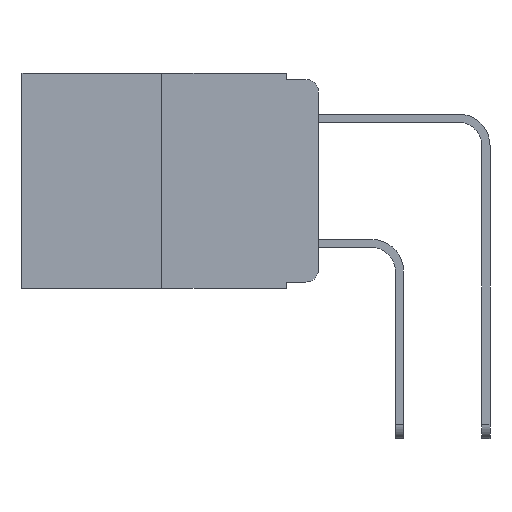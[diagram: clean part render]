
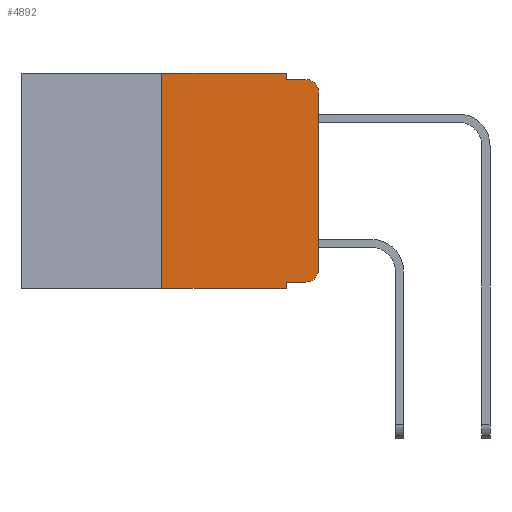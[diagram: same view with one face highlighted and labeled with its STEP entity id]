
A CAD part, left-side view. The second image highlights one B-rep face of the part: STEP entity #4892.
In plain terms, the highlighted planar face has unit normal (-1, 0, 0).
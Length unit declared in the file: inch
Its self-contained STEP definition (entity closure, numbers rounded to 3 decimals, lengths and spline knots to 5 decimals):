
#120 = LINE ( 'NONE', #3760, #2775 ) ;
#533 = VERTEX_POINT ( 'NONE', #3398 ) ;
#563 = EDGE_CURVE ( 'NONE', #5726, #13328, #4912, .T. ) ;
#716 = AXIS2_PLACEMENT_3D ( 'NONE', #894, #8579, #2016 ) ;
#840 = ORIENTED_EDGE ( 'NONE', *, *, #13257, .F. ) ;
#894 = CARTESIAN_POINT ( 'NONE',  ( 0., 0.02, -0.313 ) ) ;
#1143 = DIRECTION ( 'NONE',  ( 0., 0., -1. ) ) ;
#1167 = CARTESIAN_POINT ( 'NONE',  ( 0., 0.02, -0.01 ) ) ;
#1202 = AXIS2_PLACEMENT_3D ( 'NONE', #4929, #8517, #8490 ) ;
#1259 = ORIENTED_EDGE ( 'NONE', *, *, #12910, .F. ) ;
#1360 = VECTOR ( 'NONE', #7887, 39.37008 ) ;
#1500 = VERTEX_POINT ( 'NONE', #2942 ) ;
#1526 = FACE_OUTER_BOUND ( 'NONE', #5197, .T. ) ;
#1899 = EDGE_CURVE ( 'NONE', #3154, #9346, #120, .T. ) ;
#2016 = DIRECTION ( 'NONE',  ( 0., 0., -1. ) ) ;
#2288 = EDGE_CURVE ( 'NONE', #3154, #12996, #7619, .T. ) ;
#2687 = CARTESIAN_POINT ( 'NONE',  ( 0., 0., -0.03 ) ) ;
#2737 = CARTESIAN_POINT ( 'NONE',  ( 0., 0.02, -0.333 ) ) ;
#2763 = ORIENTED_EDGE ( 'NONE', *, *, #1899, .F. ) ;
#2775 = VECTOR ( 'NONE', #8216, 39.37008 ) ;
#2942 = CARTESIAN_POINT ( 'NONE',  ( 0., 0.051, 0. ) ) ;
#3154 = VERTEX_POINT ( 'NONE', #10959 ) ;
#3174 = VERTEX_POINT ( 'NONE', #12846 ) ;
#3245 = LINE ( 'NONE', #8955, #5864 ) ;
#3398 = CARTESIAN_POINT ( 'NONE',  ( 0., 0., -0.313 ) ) ;
#3599 = DIRECTION ( 'NONE',  ( 0., -1., 0. ) ) ;
#3760 = CARTESIAN_POINT ( 'NONE',  ( 0., 0.051, 0. ) ) ;
#3781 = CARTESIAN_POINT ( 'NONE',  ( 0., 0.25, -0.343 ) ) ;
#4087 = VERTEX_POINT ( 'NONE', #9158 ) ;
#4281 = EDGE_CURVE ( 'NONE', #8876, #3174, #3245, .T. ) ;
#4892 = ADVANCED_FACE ( 'NONE', ( #1526 ), #13605, .F. ) ;
#4912 = CIRCLE ( 'NONE', #10107, 0.02 ) ;
#4929 = CARTESIAN_POINT ( 'NONE',  ( 0., 0.473, 0. ) ) ;
#5197 = EDGE_LOOP ( 'NONE', ( #13562, #7465, #7934, #1259, #840, #12431, #11138, #2763, #11366, #8012 ) ) ;
#5726 = VERTEX_POINT ( 'NONE', #2687 ) ;
#5864 = VECTOR ( 'NONE', #13428, 39.37008 ) ;
#6359 = CARTESIAN_POINT ( 'NONE',  ( 0., 0.051, -0.01 ) ) ;
#6771 = LINE ( 'NONE', #8696, #8895 ) ;
#6962 = CIRCLE ( 'NONE', #716, 0.02 ) ;
#7018 = LINE ( 'NONE', #6359, #12185 ) ;
#7078 = DIRECTION ( 'NONE',  ( 0., -1., 0. ) ) ;
#7273 = VECTOR ( 'NONE', #3599, 39.37008 ) ;
#7463 = DIRECTION ( 'NONE',  ( 0., -1., 0. ) ) ;
#7465 = ORIENTED_EDGE ( 'NONE', *, *, #563, .T. ) ;
#7619 = LINE ( 'NONE', #13013, #7273 ) ;
#7887 = DIRECTION ( 'NONE',  ( 0., 0., 1. ) ) ;
#7934 = ORIENTED_EDGE ( 'NONE', *, *, #10855, .F. ) ;
#7939 = VECTOR ( 'NONE', #13244, 39.37008 ) ;
#8012 = ORIENTED_EDGE ( 'NONE', *, *, #12567, .T. ) ;
#8216 = DIRECTION ( 'NONE',  ( 0., 0., -1. ) ) ;
#8268 = EDGE_CURVE ( 'NONE', #8876, #9346, #12326, .T. ) ;
#8490 = DIRECTION ( 'NONE',  ( 0., 0., -1. ) ) ;
#8517 = DIRECTION ( 'NONE',  ( 1., 0., 0. ) ) ;
#8579 = DIRECTION ( 'NONE',  ( -1., 0., 0. ) ) ;
#8651 = DIRECTION ( 'NONE',  ( 0., -1., 0. ) ) ;
#8657 = DIRECTION ( 'NONE',  ( -1., 0., 0. ) ) ;
#8696 = CARTESIAN_POINT ( 'NONE',  ( 0., 0.473, 0. ) ) ;
#8876 = VERTEX_POINT ( 'NONE', #3781 ) ;
#8895 = VECTOR ( 'NONE', #8651, 39.37008 ) ;
#8955 = CARTESIAN_POINT ( 'NONE',  ( 0., 0.25, 0. ) ) ;
#9158 = CARTESIAN_POINT ( 'NONE',  ( 0., 0.051, -0.01 ) ) ;
#9346 = VERTEX_POINT ( 'NONE', #13004 ) ;
#9581 = VECTOR ( 'NONE', #7078, 39.37008 ) ;
#10107 = AXIS2_PLACEMENT_3D ( 'NONE', #12541, #8657, #1143 ) ;
#10855 = EDGE_CURVE ( 'NONE', #4087, #13328, #7018, .T. ) ;
#10959 = CARTESIAN_POINT ( 'NONE',  ( 0., 0.051, -0.333 ) ) ;
#11138 = ORIENTED_EDGE ( 'NONE', *, *, #8268, .T. ) ;
#11158 = CARTESIAN_POINT ( 'NONE',  ( 0., 0.051, 0. ) ) ;
#11164 = CARTESIAN_POINT ( 'NONE',  ( 0., 0.473, -0.343 ) ) ;
#11366 = ORIENTED_EDGE ( 'NONE', *, *, #2288, .T. ) ;
#12185 = VECTOR ( 'NONE', #7463, 39.37008 ) ;
#12326 = LINE ( 'NONE', #11164, #9581 ) ;
#12431 = ORIENTED_EDGE ( 'NONE', *, *, #4281, .F. ) ;
#12541 = CARTESIAN_POINT ( 'NONE',  ( 0., 0.02, -0.03 ) ) ;
#12567 = EDGE_CURVE ( 'NONE', #12996, #533, #6962, .T. ) ;
#12748 = LINE ( 'NONE', #13015, #1360 ) ;
#12846 = CARTESIAN_POINT ( 'NONE',  ( 0., 0.25, 0. ) ) ;
#12910 = EDGE_CURVE ( 'NONE', #1500, #4087, #13388, .T. ) ;
#12996 = VERTEX_POINT ( 'NONE', #2737 ) ;
#13004 = CARTESIAN_POINT ( 'NONE',  ( 0., 0.051, -0.343 ) ) ;
#13013 = CARTESIAN_POINT ( 'NONE',  ( 0., 0.051, -0.333 ) ) ;
#13015 = CARTESIAN_POINT ( 'NONE',  ( 0., 0., 0. ) ) ;
#13244 = DIRECTION ( 'NONE',  ( 0., 0., -1. ) ) ;
#13257 = EDGE_CURVE ( 'NONE', #3174, #1500, #6771, .T. ) ;
#13328 = VERTEX_POINT ( 'NONE', #1167 ) ;
#13376 = EDGE_CURVE ( 'NONE', #533, #5726, #12748, .T. ) ;
#13388 = LINE ( 'NONE', #11158, #7939 ) ;
#13428 = DIRECTION ( 'NONE',  ( 0., 0., 1. ) ) ;
#13562 = ORIENTED_EDGE ( 'NONE', *, *, #13376, .T. ) ;
#13605 = PLANE ( 'NONE',  #1202 ) ;
